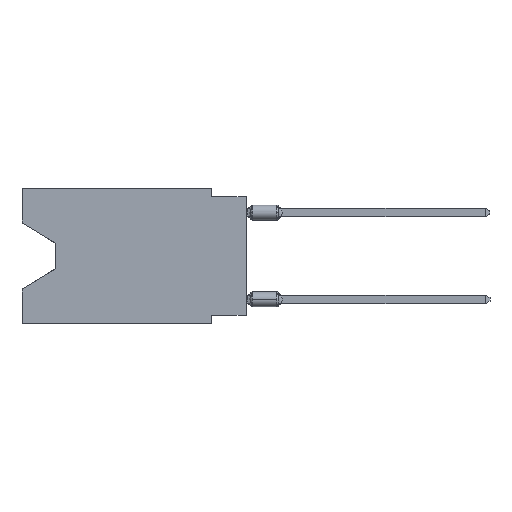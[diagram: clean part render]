
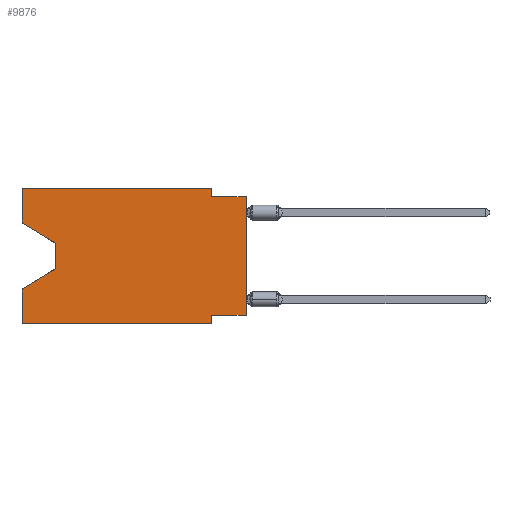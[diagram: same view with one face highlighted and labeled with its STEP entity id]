
A CAD part, left-side view. The second image highlights one B-rep face of the part: STEP entity #9876.
In plain terms, the highlighted planar face has unit normal (-1, 0, 0).
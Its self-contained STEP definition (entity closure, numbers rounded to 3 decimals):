
#193 = LINE ( 'NONE', #5791, #13790 ) ;
#491 = EDGE_CURVE ( 'NONE', #1392, #7484, #13883, .T. ) ;
#522 = EDGE_CURVE ( 'NONE', #12402, #7484, #4288, .T. ) ;
#789 = VERTEX_POINT ( 'NONE', #3488 ) ;
#1183 = LINE ( 'NONE', #5620, #6828 ) ;
#1256 = EDGE_CURVE ( 'NONE', #9725, #4568, #3321, .T. ) ;
#1283 = CARTESIAN_POINT ( 'NONE',  ( 0., 0., -9.271 ) ) ;
#1345 = CARTESIAN_POINT ( 'NONE',  ( 0., 13.97, -5.893 ) ) ;
#1375 = DIRECTION ( 'NONE',  ( 0., 0., 1. ) ) ;
#1392 = VERTEX_POINT ( 'NONE', #4028 ) ;
#2108 = LINE ( 'NONE', #6546, #6082 ) ;
#2495 = ORIENTED_EDGE ( 'NONE', *, *, #7710, .F. ) ;
#2680 = ORIENTED_EDGE ( 'NONE', *, *, #11780, .T. ) ;
#2911 = AXIS2_PLACEMENT_3D ( 'NONE', #13196, #13120, #5546 ) ;
#2975 = ORIENTED_EDGE ( 'NONE', *, *, #11012, .F. ) ;
#3049 = CARTESIAN_POINT ( 'NONE',  ( 0., 16.383, -9.906 ) ) ;
#3321 = LINE ( 'NONE', #10008, #5747 ) ;
#3488 = CARTESIAN_POINT ( 'NONE',  ( 0., 2.54, -0.635 ) ) ;
#3595 = ORIENTED_EDGE ( 'NONE', *, *, #11383, .F. ) ;
#3785 = CARTESIAN_POINT ( 'NONE',  ( 0., 2.54, 0. ) ) ;
#4028 = CARTESIAN_POINT ( 'NONE',  ( 0., 2.54, -9.271 ) ) ;
#4101 = VECTOR ( 'NONE', #13672, 1000. ) ;
#4124 = CARTESIAN_POINT ( 'NONE',  ( 0., 2.54, 0. ) ) ;
#4185 = DIRECTION ( 'NONE',  ( 0., 0., -1. ) ) ;
#4261 = CARTESIAN_POINT ( 'NONE',  ( 0., 13.97, -4.013 ) ) ;
#4288 = LINE ( 'NONE', #13164, #9918 ) ;
#4361 = ORIENTED_EDGE ( 'NONE', *, *, #10533, .F. ) ;
#4482 = DIRECTION ( 'NONE',  ( 0., -1., 0. ) ) ;
#4568 = VERTEX_POINT ( 'NONE', #4124 ) ;
#4880 = DIRECTION ( 'NONE',  ( 0., 0., 1. ) ) ;
#5082 = DIRECTION ( 'NONE',  ( 0., 0., -1. ) ) ;
#5096 = ORIENTED_EDGE ( 'NONE', *, *, #522, .T. ) ;
#5138 = VECTOR ( 'NONE', #1375, 1000. ) ;
#5221 = VERTEX_POINT ( 'NONE', #6940 ) ;
#5496 = ORIENTED_EDGE ( 'NONE', *, *, #6195, .T. ) ;
#5502 = VERTEX_POINT ( 'NONE', #6629 ) ;
#5546 = DIRECTION ( 'NONE',  ( 0., 0., -1. ) ) ;
#5620 = CARTESIAN_POINT ( 'NONE',  ( 0., 0., 0. ) ) ;
#5747 = VECTOR ( 'NONE', #4482, 1000. ) ;
#5791 = CARTESIAN_POINT ( 'NONE',  ( 0., 0., -9.271 ) ) ;
#6082 = VECTOR ( 'NONE', #11058, 1000. ) ;
#6195 = EDGE_CURVE ( 'NONE', #10965, #5221, #6360, .T. ) ;
#6284 = CARTESIAN_POINT ( 'NONE',  ( 0., 16.383, -2.546 ) ) ;
#6360 = LINE ( 'NONE', #4261, #10953 ) ;
#6546 = CARTESIAN_POINT ( 'NONE',  ( 0., 16.383, -2.546 ) ) ;
#6629 = CARTESIAN_POINT ( 'NONE',  ( 0., 0., -0.635 ) ) ;
#6828 = VECTOR ( 'NONE', #8031, 1000. ) ;
#6923 = CARTESIAN_POINT ( 'NONE',  ( 0., 13.97, -4.013 ) ) ;
#6940 = CARTESIAN_POINT ( 'NONE',  ( 0., 13.97, -5.893 ) ) ;
#7242 = ORIENTED_EDGE ( 'NONE', *, *, #8572, .T. ) ;
#7443 = CARTESIAN_POINT ( 'NONE',  ( 0., 16.383, 0. ) ) ;
#7484 = VERTEX_POINT ( 'NONE', #12688 ) ;
#7641 = EDGE_LOOP ( 'NONE', ( #8798, #5496, #7242, #2495, #5096, #7713, #3595, #2680, #10847, #4361, #10513, #2975 ) ) ;
#7707 = CARTESIAN_POINT ( 'NONE',  ( 0., 16.383, -7.36 ) ) ;
#7710 = EDGE_CURVE ( 'NONE', #12402, #12419, #14048, .T. ) ;
#7713 = ORIENTED_EDGE ( 'NONE', *, *, #491, .F. ) ;
#8031 = DIRECTION ( 'NONE',  ( 0., 0., 1. ) ) ;
#8535 = CARTESIAN_POINT ( 'NONE',  ( 0., 16.383, 0. ) ) ;
#8572 = EDGE_CURVE ( 'NONE', #5221, #12419, #10148, .T. ) ;
#8798 = ORIENTED_EDGE ( 'NONE', *, *, #9124, .T. ) ;
#9124 = EDGE_CURVE ( 'NONE', #11451, #10965, #2108, .T. ) ;
#9324 = CARTESIAN_POINT ( 'NONE',  ( 0., 16.383, 0. ) ) ;
#9725 = VERTEX_POINT ( 'NONE', #7443 ) ;
#9876 = ADVANCED_FACE ( 'NONE', ( #12107 ), #12037, .F. ) ;
#9918 = VECTOR ( 'NONE', #10614, 1000. ) ;
#10008 = CARTESIAN_POINT ( 'NONE',  ( 0., 16.383, 0. ) ) ;
#10148 = LINE ( 'NONE', #1345, #12585 ) ;
#10233 = DIRECTION ( 'NONE',  ( 0., 1., 0. ) ) ;
#10340 = LINE ( 'NONE', #9324, #13381 ) ;
#10513 = ORIENTED_EDGE ( 'NONE', *, *, #1256, .F. ) ;
#10533 = EDGE_CURVE ( 'NONE', #4568, #789, #11695, .T. ) ;
#10614 = DIRECTION ( 'NONE',  ( 0., -1., 0. ) ) ;
#10706 = EDGE_CURVE ( 'NONE', #789, #5502, #14167, .T. ) ;
#10847 = ORIENTED_EDGE ( 'NONE', *, *, #10706, .F. ) ;
#10953 = VECTOR ( 'NONE', #4185, 1000. ) ;
#10965 = VERTEX_POINT ( 'NONE', #6923 ) ;
#11012 = EDGE_CURVE ( 'NONE', #11451, #9725, #10340, .T. ) ;
#11046 = VECTOR ( 'NONE', #5082, 1000. ) ;
#11058 = DIRECTION ( 'NONE',  ( 0., -0.855, -0.519 ) ) ;
#11278 = VERTEX_POINT ( 'NONE', #1283 ) ;
#11383 = EDGE_CURVE ( 'NONE', #11278, #1392, #193, .T. ) ;
#11451 = VERTEX_POINT ( 'NONE', #6284 ) ;
#11629 = CARTESIAN_POINT ( 'NONE',  ( 0., 2.54, -9.906 ) ) ;
#11695 = LINE ( 'NONE', #3785, #11046 ) ;
#11780 = EDGE_CURVE ( 'NONE', #11278, #5502, #1183, .T. ) ;
#11863 = DIRECTION ( 'NONE',  ( 0., -1., 0. ) ) ;
#12001 = VECTOR ( 'NONE', #11863, 1000. ) ;
#12037 = PLANE ( 'NONE',  #2911 ) ;
#12107 = FACE_OUTER_BOUND ( 'NONE', #7641, .T. ) ;
#12402 = VERTEX_POINT ( 'NONE', #3049 ) ;
#12419 = VERTEX_POINT ( 'NONE', #7707 ) ;
#12585 = VECTOR ( 'NONE', #13629, 1000. ) ;
#12688 = CARTESIAN_POINT ( 'NONE',  ( 0., 2.54, -9.906 ) ) ;
#13086 = CARTESIAN_POINT ( 'NONE',  ( 0., 0., -0.635 ) ) ;
#13120 = DIRECTION ( 'NONE',  ( 1., 0., 0. ) ) ;
#13164 = CARTESIAN_POINT ( 'NONE',  ( 0., 16.383, -9.906 ) ) ;
#13196 = CARTESIAN_POINT ( 'NONE',  ( 0., 16.383, 0. ) ) ;
#13381 = VECTOR ( 'NONE', #4880, 1000. ) ;
#13629 = DIRECTION ( 'NONE',  ( 0., 0.855, -0.519 ) ) ;
#13672 = DIRECTION ( 'NONE',  ( 0., 0., -1. ) ) ;
#13790 = VECTOR ( 'NONE', #10233, 1000. ) ;
#13883 = LINE ( 'NONE', #11629, #4101 ) ;
#14048 = LINE ( 'NONE', #8535, #5138 ) ;
#14167 = LINE ( 'NONE', #13086, #12001 ) ;
